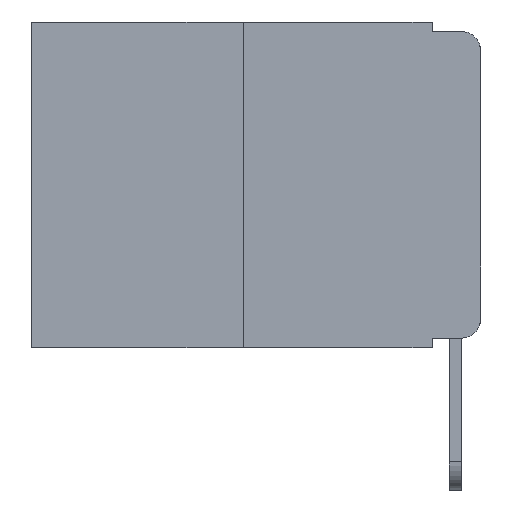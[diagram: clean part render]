
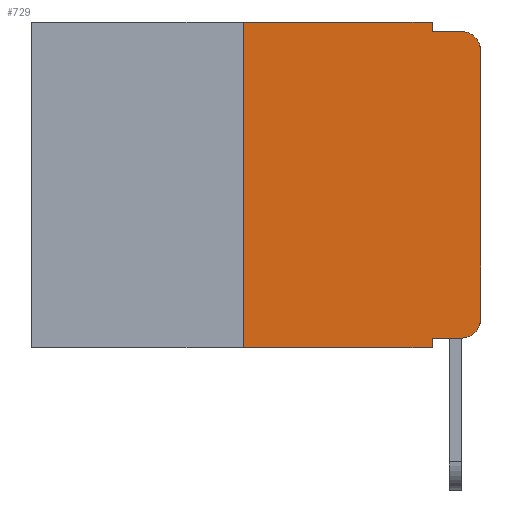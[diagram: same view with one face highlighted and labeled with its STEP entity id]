
A CAD part, left-side view. The second image highlights one B-rep face of the part: STEP entity #729.
In plain terms, the highlighted planar face has unit normal (-1, 0, 0).
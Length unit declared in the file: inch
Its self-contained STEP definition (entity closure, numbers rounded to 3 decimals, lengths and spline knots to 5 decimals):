
#136 = VECTOR ( 'NONE', #5577, 39.37008 ) ;
#198 = ORIENTED_EDGE ( 'NONE', *, *, #10483, .T. ) ;
#229 = VERTEX_POINT ( 'NONE', #9004 ) ;
#529 = VECTOR ( 'NONE', #11263, 39.37008 ) ;
#729 = ADVANCED_FACE ( 'NONE', ( #2251 ), #5432, .F. ) ;
#787 = CARTESIAN_POINT ( 'NONE',  ( 0., 0.473, -0.343 ) ) ;
#860 = VERTEX_POINT ( 'NONE', #1034 ) ;
#1034 = CARTESIAN_POINT ( 'NONE',  ( 0., 0.25, 0. ) ) ;
#1071 = CARTESIAN_POINT ( 'NONE',  ( 0., 0.051, 0. ) ) ;
#1263 = ORIENTED_EDGE ( 'NONE', *, *, #7700, .T. ) ;
#1362 = DIRECTION ( 'NONE',  ( -1., 0., 0. ) ) ;
#1400 = ORIENTED_EDGE ( 'NONE', *, *, #13587, .F. ) ;
#1526 = EDGE_CURVE ( 'NONE', #11760, #860, #9146, .T. ) ;
#1683 = VERTEX_POINT ( 'NONE', #1071 ) ;
#1706 = VECTOR ( 'NONE', #4103, 39.37008 ) ;
#1892 = CARTESIAN_POINT ( 'NONE',  ( 0., 0.051, -0.333 ) ) ;
#2237 = VERTEX_POINT ( 'NONE', #3339 ) ;
#2251 = FACE_OUTER_BOUND ( 'NONE', #9427, .T. ) ;
#2261 = CARTESIAN_POINT ( 'NONE',  ( 0., 0.051, 0. ) ) ;
#2933 = CARTESIAN_POINT ( 'NONE',  ( 0., 0.25, 0. ) ) ;
#2941 = DIRECTION ( 'NONE',  ( 0., -1., 0. ) ) ;
#3008 = CARTESIAN_POINT ( 'NONE',  ( 0., 0.473, 0. ) ) ;
#3027 = EDGE_CURVE ( 'NONE', #4012, #229, #5733, .T. ) ;
#3194 = CARTESIAN_POINT ( 'NONE',  ( 0., 0., -0.313 ) ) ;
#3339 = CARTESIAN_POINT ( 'NONE',  ( 0., 0.051, -0.343 ) ) ;
#3587 = EDGE_CURVE ( 'NONE', #8683, #2237, #3812, .T. ) ;
#3812 = LINE ( 'NONE', #3951, #8167 ) ;
#3951 = CARTESIAN_POINT ( 'NONE',  ( 0., 0.051, 0. ) ) ;
#4012 = VERTEX_POINT ( 'NONE', #12268 ) ;
#4027 = AXIS2_PLACEMENT_3D ( 'NONE', #10983, #1362, #5672 ) ;
#4103 = DIRECTION ( 'NONE',  ( 0., -1., 0. ) ) ;
#4410 = AXIS2_PLACEMENT_3D ( 'NONE', #5666, #11762, #6625 ) ;
#4946 = AXIS2_PLACEMENT_3D ( 'NONE', #7497, #11800, #6462 ) ;
#5115 = LINE ( 'NONE', #12599, #12400 ) ;
#5432 = PLANE ( 'NONE',  #4946 ) ;
#5577 = DIRECTION ( 'NONE',  ( 0., 0., -1. ) ) ;
#5666 = CARTESIAN_POINT ( 'NONE',  ( 0., 0.02, -0.313 ) ) ;
#5672 = DIRECTION ( 'NONE',  ( 0., 0., -1. ) ) ;
#5733 = LINE ( 'NONE', #9981, #13260 ) ;
#5977 = VECTOR ( 'NONE', #12592, 39.37008 ) ;
#6225 = DIRECTION ( 'NONE',  ( 0., 0., 1. ) ) ;
#6234 = CARTESIAN_POINT ( 'NONE',  ( 0., 0.051, -0.333 ) ) ;
#6295 = EDGE_CURVE ( 'NONE', #13677, #229, #10043, .T. ) ;
#6462 = DIRECTION ( 'NONE',  ( 0., 0., -1. ) ) ;
#6625 = DIRECTION ( 'NONE',  ( 0., 0., -1. ) ) ;
#6794 = ORIENTED_EDGE ( 'NONE', *, *, #1526, .F. ) ;
#6812 = CARTESIAN_POINT ( 'NONE',  ( 0., 0., -0.03 ) ) ;
#6970 = VERTEX_POINT ( 'NONE', #3194 ) ;
#7048 = LINE ( 'NONE', #3008, #12507 ) ;
#7207 = CARTESIAN_POINT ( 'NONE',  ( 0., 0.25, -0.343 ) ) ;
#7497 = CARTESIAN_POINT ( 'NONE',  ( 0., 0.473, 0. ) ) ;
#7502 = VERTEX_POINT ( 'NONE', #10074 ) ;
#7671 = ORIENTED_EDGE ( 'NONE', *, *, #10790, .T. ) ;
#7700 = EDGE_CURVE ( 'NONE', #6970, #13677, #5115, .T. ) ;
#8068 = DIRECTION ( 'NONE',  ( 0., 0., -1. ) ) ;
#8167 = VECTOR ( 'NONE', #8068, 39.37008 ) ;
#8362 = ORIENTED_EDGE ( 'NONE', *, *, #6295, .T. ) ;
#8683 = VERTEX_POINT ( 'NONE', #6234 ) ;
#8728 = DIRECTION ( 'NONE',  ( 0., -1., 0. ) ) ;
#8789 = ORIENTED_EDGE ( 'NONE', *, *, #3587, .F. ) ;
#9004 = CARTESIAN_POINT ( 'NONE',  ( 0., 0.02, -0.01 ) ) ;
#9146 = LINE ( 'NONE', #2933, #529 ) ;
#9323 = EDGE_CURVE ( 'NONE', #7502, #6970, #9514, .T. ) ;
#9427 = EDGE_LOOP ( 'NONE', ( #1263, #8362, #12187, #10607, #1400, #6794, #198, #8789, #7671, #10757 ) ) ;
#9514 = CIRCLE ( 'NONE', #4410, 0.02 ) ;
#9981 = CARTESIAN_POINT ( 'NONE',  ( 0., 0.051, -0.01 ) ) ;
#10043 = CIRCLE ( 'NONE', #4027, 0.02 ) ;
#10074 = CARTESIAN_POINT ( 'NONE',  ( 0., 0.02, -0.333 ) ) ;
#10405 = LINE ( 'NONE', #787, #5977 ) ;
#10483 = EDGE_CURVE ( 'NONE', #11760, #2237, #10405, .T. ) ;
#10607 = ORIENTED_EDGE ( 'NONE', *, *, #12922, .F. ) ;
#10757 = ORIENTED_EDGE ( 'NONE', *, *, #9323, .T. ) ;
#10790 = EDGE_CURVE ( 'NONE', #8683, #7502, #13697, .T. ) ;
#10983 = CARTESIAN_POINT ( 'NONE',  ( 0., 0.02, -0.03 ) ) ;
#11263 = DIRECTION ( 'NONE',  ( 0., 0., 1. ) ) ;
#11760 = VERTEX_POINT ( 'NONE', #7207 ) ;
#11762 = DIRECTION ( 'NONE',  ( -1., 0., 0. ) ) ;
#11800 = DIRECTION ( 'NONE',  ( 1., 0., 0. ) ) ;
#11882 = LINE ( 'NONE', #2261, #136 ) ;
#12187 = ORIENTED_EDGE ( 'NONE', *, *, #3027, .F. ) ;
#12268 = CARTESIAN_POINT ( 'NONE',  ( 0., 0.051, -0.01 ) ) ;
#12400 = VECTOR ( 'NONE', #6225, 39.37008 ) ;
#12507 = VECTOR ( 'NONE', #2941, 39.37008 ) ;
#12592 = DIRECTION ( 'NONE',  ( 0., -1., 0. ) ) ;
#12599 = CARTESIAN_POINT ( 'NONE',  ( 0., 0., 0. ) ) ;
#12922 = EDGE_CURVE ( 'NONE', #1683, #4012, #11882, .T. ) ;
#13260 = VECTOR ( 'NONE', #8728, 39.37008 ) ;
#13587 = EDGE_CURVE ( 'NONE', #860, #1683, #7048, .T. ) ;
#13677 = VERTEX_POINT ( 'NONE', #6812 ) ;
#13697 = LINE ( 'NONE', #1892, #1706 ) ;
